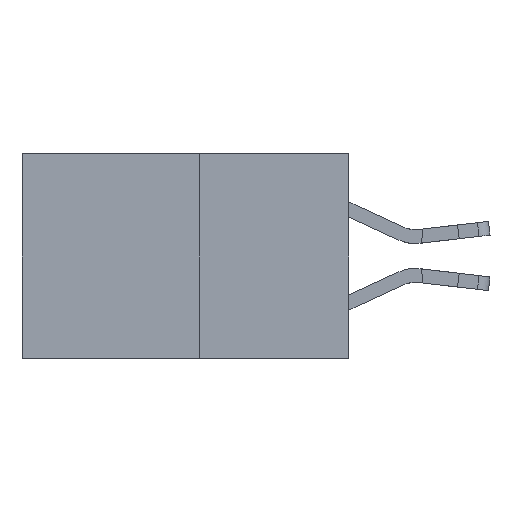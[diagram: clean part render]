
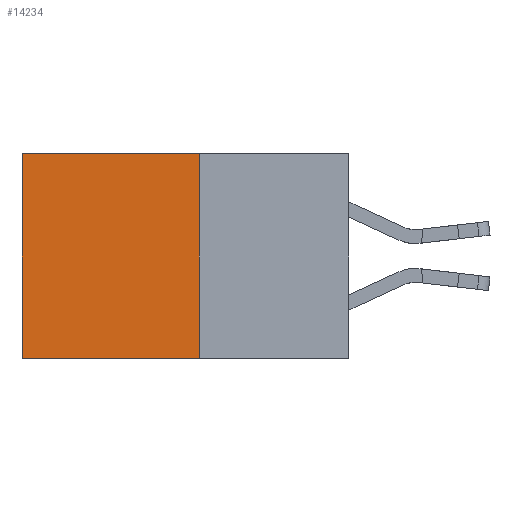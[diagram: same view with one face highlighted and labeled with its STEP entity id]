
A CAD part, left-side view. The second image highlights one B-rep face of the part: STEP entity #14234.
In plain terms, the highlighted planar face has unit normal (-1, 0, 0).
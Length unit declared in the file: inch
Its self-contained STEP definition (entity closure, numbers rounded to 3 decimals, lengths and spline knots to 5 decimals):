
#991 = DIRECTION ( 'NONE',  ( 0., 0., -1. ) ) ;
#1144 = LINE ( 'NONE', #22996, #11217 ) ;
#1806 = LINE ( 'NONE', #2218, #16082 ) ;
#2218 = CARTESIAN_POINT ( 'NONE',  ( 0.277, 0.27, 0. ) ) ;
#2779 = VERTEX_POINT ( 'NONE', #5990 ) ;
#2979 = VECTOR ( 'NONE', #17447, 39.37008 ) ;
#4513 = ORIENTED_EDGE ( 'NONE', *, *, #6516, .F. ) ;
#5541 = EDGE_CURVE ( 'NONE', #13005, #16445, #12979, .T. ) ;
#5583 = EDGE_CURVE ( 'NONE', #2779, #20334, #1806, .T. ) ;
#5990 = CARTESIAN_POINT ( 'NONE',  ( 0.277, 0.27, 0. ) ) ;
#6058 = CARTESIAN_POINT ( 'NONE',  ( 0.277, 0.59, 0. ) ) ;
#6415 = EDGE_CURVE ( 'NONE', #20334, #16445, #17748, .T. ) ;
#6516 = EDGE_CURVE ( 'NONE', #2779, #13005, #1144, .T. ) ;
#7474 = PLANE ( 'NONE',  #16966 ) ;
#7775 = CARTESIAN_POINT ( 'NONE',  ( 0.277, 0.27, -0.37 ) ) ;
#8764 = ORIENTED_EDGE ( 'NONE', *, *, #5583, .T. ) ;
#11217 = VECTOR ( 'NONE', #991, 39.37008 ) ;
#11221 = DIRECTION ( 'NONE',  ( 1., 0., 0. ) ) ;
#11364 = FACE_OUTER_BOUND ( 'NONE', #22482, .T. ) ;
#12979 = LINE ( 'NONE', #7775, #22463 ) ;
#13005 = VERTEX_POINT ( 'NONE', #20795 ) ;
#13757 = CARTESIAN_POINT ( 'NONE',  ( 0.277, 0.59, -0.37 ) ) ;
#14234 = ADVANCED_FACE ( 'NONE', ( #11364 ), #7474, .F. ) ;
#15114 = DIRECTION ( 'NONE',  ( 0., 1., 0. ) ) ;
#16082 = VECTOR ( 'NONE', #20628, 39.37008 ) ;
#16445 = VERTEX_POINT ( 'NONE', #20919 ) ;
#16966 = AXIS2_PLACEMENT_3D ( 'NONE', #23656, #11221, #23735 ) ;
#17447 = DIRECTION ( 'NONE',  ( 0., 0., -1. ) ) ;
#17748 = LINE ( 'NONE', #13757, #2979 ) ;
#20334 = VERTEX_POINT ( 'NONE', #6058 ) ;
#20628 = DIRECTION ( 'NONE',  ( 0., 1., 0. ) ) ;
#20795 = CARTESIAN_POINT ( 'NONE',  ( 0.277, 0.27, -0.37 ) ) ;
#20919 = CARTESIAN_POINT ( 'NONE',  ( 0.277, 0.59, -0.37 ) ) ;
#22463 = VECTOR ( 'NONE', #15114, 39.37008 ) ;
#22482 = EDGE_LOOP ( 'NONE', ( #23653, #23237, #4513, #8764 ) ) ;
#22996 = CARTESIAN_POINT ( 'NONE',  ( 0.277, 0.27, -0.37 ) ) ;
#23237 = ORIENTED_EDGE ( 'NONE', *, *, #5541, .F. ) ;
#23653 = ORIENTED_EDGE ( 'NONE', *, *, #6415, .T. ) ;
#23656 = CARTESIAN_POINT ( 'NONE',  ( 0.277, 0.27, -0.37 ) ) ;
#23735 = DIRECTION ( 'NONE',  ( 0., 0., -1. ) ) ;
